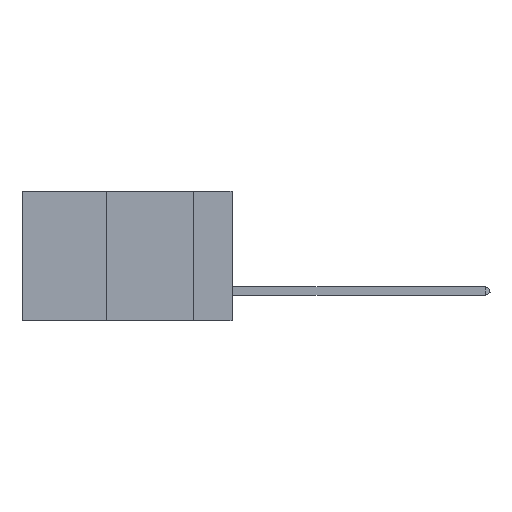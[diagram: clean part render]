
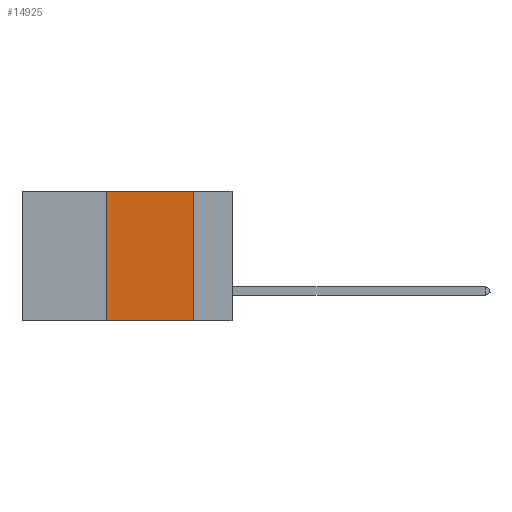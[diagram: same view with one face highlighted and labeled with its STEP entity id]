
A CAD part, left-side view. The second image highlights one B-rep face of the part: STEP entity #14925.
In plain terms, the highlighted planar face has unit normal (-1, 0, 0).
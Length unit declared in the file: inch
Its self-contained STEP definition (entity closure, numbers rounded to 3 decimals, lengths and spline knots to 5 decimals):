
#626 = VECTOR ( 'NONE', #12757, 39.37008 ) ;
#1470 = VECTOR ( 'NONE', #14450, 39.37008 ) ;
#1505 = CARTESIAN_POINT ( 'NONE',  ( 0., 0.36, 0. ) ) ;
#2086 = CARTESIAN_POINT ( 'NONE',  ( 0., 0.11, -0.37 ) ) ;
#2316 = EDGE_CURVE ( 'NONE', #17569, #17535, #10371, .T. ) ;
#2322 = ORIENTED_EDGE ( 'NONE', *, *, #4428, .T. ) ;
#2723 = DIRECTION ( 'NONE',  ( 0., 0., -1. ) ) ;
#3604 = EDGE_CURVE ( 'NONE', #18202, #17569, #14973, .T. ) ;
#4428 = EDGE_CURVE ( 'NONE', #18202, #9118, #14407, .T. ) ;
#7065 = CARTESIAN_POINT ( 'NONE',  ( 0., 0.6, -0.37 ) ) ;
#8136 = CARTESIAN_POINT ( 'NONE',  ( 0., 0.11, 0. ) ) ;
#8375 = EDGE_CURVE ( 'NONE', #17535, #9118, #12020, .T. ) ;
#8988 = DIRECTION ( 'NONE',  ( 0., 0., -1. ) ) ;
#9061 = CARTESIAN_POINT ( 'NONE',  ( 0., 0.6, 0. ) ) ;
#9118 = VERTEX_POINT ( 'NONE', #2086 ) ;
#9741 = VECTOR ( 'NONE', #2723, 39.37008 ) ;
#10371 = LINE ( 'NONE', #21014, #1470 ) ;
#10421 = ORIENTED_EDGE ( 'NONE', *, *, #2316, .F. ) ;
#10620 = DIRECTION ( 'NONE',  ( 1., 0., 0. ) ) ;
#10710 = CARTESIAN_POINT ( 'NONE',  ( 0., 0.11, 0. ) ) ;
#12020 = LINE ( 'NONE', #10710, #9741 ) ;
#12757 = DIRECTION ( 'NONE',  ( 0., 0., 1. ) ) ;
#13624 = CARTESIAN_POINT ( 'NONE',  ( 0., 0.36, 0. ) ) ;
#14407 = LINE ( 'NONE', #7065, #19325 ) ;
#14450 = DIRECTION ( 'NONE',  ( 0., -1., 0. ) ) ;
#14712 = AXIS2_PLACEMENT_3D ( 'NONE', #9061, #10620, #8988 ) ;
#14925 = ADVANCED_FACE ( 'NONE', ( #18306 ), #19090, .F. ) ;
#14973 = LINE ( 'NONE', #13624, #626 ) ;
#15523 = DIRECTION ( 'NONE',  ( 0., -1., 0. ) ) ;
#16515 = CARTESIAN_POINT ( 'NONE',  ( 0., 0.36, -0.37 ) ) ;
#17535 = VERTEX_POINT ( 'NONE', #8136 ) ;
#17569 = VERTEX_POINT ( 'NONE', #1505 ) ;
#18202 = VERTEX_POINT ( 'NONE', #16515 ) ;
#18306 = FACE_OUTER_BOUND ( 'NONE', #18430, .T. ) ;
#18430 = EDGE_LOOP ( 'NONE', ( #20370, #10421, #18923, #2322 ) ) ;
#18923 = ORIENTED_EDGE ( 'NONE', *, *, #3604, .F. ) ;
#19090 = PLANE ( 'NONE',  #14712 ) ;
#19325 = VECTOR ( 'NONE', #15523, 39.37008 ) ;
#20370 = ORIENTED_EDGE ( 'NONE', *, *, #8375, .F. ) ;
#21014 = CARTESIAN_POINT ( 'NONE',  ( 0., 0.6, 0. ) ) ;
